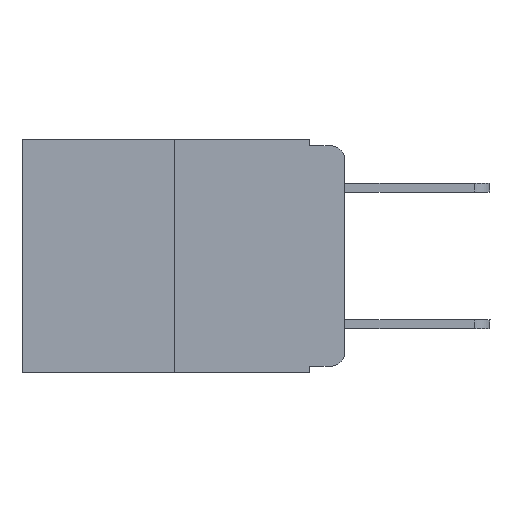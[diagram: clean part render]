
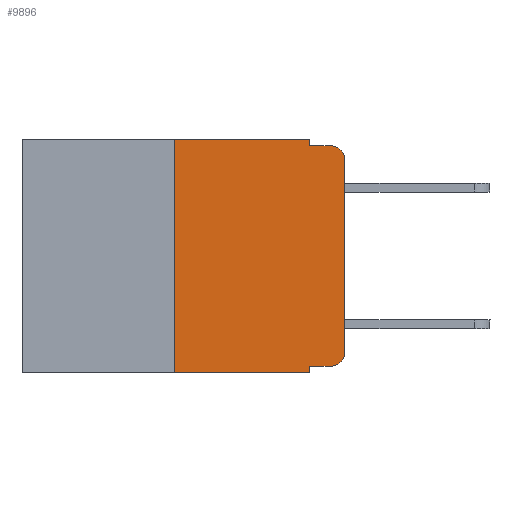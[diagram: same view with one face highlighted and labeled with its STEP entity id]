
A CAD part, left-side view. The second image highlights one B-rep face of the part: STEP entity #9896.
In plain terms, the highlighted planar face has unit normal (-1, 0, 0).
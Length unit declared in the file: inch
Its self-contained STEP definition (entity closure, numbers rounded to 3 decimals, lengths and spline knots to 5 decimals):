
#275 = LINE ( 'NONE', #21118, #16791 ) ;
#356 = DIRECTION ( 'NONE',  ( -1., 0., 0. ) ) ;
#552 = EDGE_CURVE ( 'NONE', #11415, #7567, #9098, .T. ) ;
#664 = DIRECTION ( 'NONE',  ( -1., 0., 0. ) ) ;
#775 = VERTEX_POINT ( 'NONE', #5129 ) ;
#997 = AXIS2_PLACEMENT_3D ( 'NONE', #3236, #20541, #8429 ) ;
#1747 = CARTESIAN_POINT ( 'NONE',  ( 0., 0., 0. ) ) ;
#1887 = DIRECTION ( 'NONE',  ( 0., 0., -1. ) ) ;
#2040 = VERTEX_POINT ( 'NONE', #16216 ) ;
#2120 = ORIENTED_EDGE ( 'NONE', *, *, #552, .T. ) ;
#2182 = CARTESIAN_POINT ( 'NONE',  ( 0., 0.473, -0.343 ) ) ;
#2504 = ORIENTED_EDGE ( 'NONE', *, *, #9815, .F. ) ;
#2686 = VECTOR ( 'NONE', #15383, 39.37008 ) ;
#2992 = CARTESIAN_POINT ( 'NONE',  ( 0., 0.473, 0. ) ) ;
#3052 = CARTESIAN_POINT ( 'NONE',  ( 0., 0.051, -0.01 ) ) ;
#3236 = CARTESIAN_POINT ( 'NONE',  ( 0., 0.473, 0. ) ) ;
#3288 = CARTESIAN_POINT ( 'NONE',  ( 0., 0.02, -0.333 ) ) ;
#3458 = VERTEX_POINT ( 'NONE', #17536 ) ;
#3771 = ORIENTED_EDGE ( 'NONE', *, *, #14911, .F. ) ;
#5129 = CARTESIAN_POINT ( 'NONE',  ( 0., 0.25, -0.343 ) ) ;
#5408 = VERTEX_POINT ( 'NONE', #13309 ) ;
#5728 = DIRECTION ( 'NONE',  ( 0., -1., 0. ) ) ;
#5820 = VECTOR ( 'NONE', #12043, 39.37008 ) ;
#6026 = ORIENTED_EDGE ( 'NONE', *, *, #7928, .T. ) ;
#7440 = DIRECTION ( 'NONE',  ( 0., 0., -1. ) ) ;
#7567 = VERTEX_POINT ( 'NONE', #14867 ) ;
#7669 = ORIENTED_EDGE ( 'NONE', *, *, #17644, .F. ) ;
#7928 = EDGE_CURVE ( 'NONE', #775, #10947, #13786, .T. ) ;
#8265 = CARTESIAN_POINT ( 'NONE',  ( 0., 0.051, 0. ) ) ;
#8429 = DIRECTION ( 'NONE',  ( 0., 0., -1. ) ) ;
#8486 = ORIENTED_EDGE ( 'NONE', *, *, #16528, .T. ) ;
#9098 = CIRCLE ( 'NONE', #13086, 0.02 ) ;
#9815 = EDGE_CURVE ( 'NONE', #775, #2040, #20059, .T. ) ;
#9896 = ADVANCED_FACE ( 'NONE', ( #22265 ), #11975, .F. ) ;
#10947 = VERTEX_POINT ( 'NONE', #14468 ) ;
#11323 = VECTOR ( 'NONE', #14043, 39.37008 ) ;
#11415 = VERTEX_POINT ( 'NONE', #14407 ) ;
#11485 = DIRECTION ( 'NONE',  ( 0., 0., -1. ) ) ;
#11516 = CARTESIAN_POINT ( 'NONE',  ( 0., 0.25, 0. ) ) ;
#11975 = PLANE ( 'NONE',  #997 ) ;
#12043 = DIRECTION ( 'NONE',  ( 0., 0., -1. ) ) ;
#12186 = VECTOR ( 'NONE', #5728, 39.37008 ) ;
#12619 = DIRECTION ( 'NONE',  ( 0., -1., 0. ) ) ;
#12682 = LINE ( 'NONE', #1747, #11323 ) ;
#12960 = ORIENTED_EDGE ( 'NONE', *, *, #16557, .T. ) ;
#13086 = AXIS2_PLACEMENT_3D ( 'NONE', #14498, #356, #1887 ) ;
#13309 = CARTESIAN_POINT ( 'NONE',  ( 0., 0.051, -0.01 ) ) ;
#13405 = DIRECTION ( 'NONE',  ( 0., 0., 1. ) ) ;
#13537 = VERTEX_POINT ( 'NONE', #20638 ) ;
#13786 = LINE ( 'NONE', #2182, #12186 ) ;
#13906 = CARTESIAN_POINT ( 'NONE',  ( 0., 0., -0.313 ) ) ;
#14043 = DIRECTION ( 'NONE',  ( 0., 0., 1. ) ) ;
#14078 = ORIENTED_EDGE ( 'NONE', *, *, #16243, .F. ) ;
#14108 = VECTOR ( 'NONE', #11485, 39.37008 ) ;
#14407 = CARTESIAN_POINT ( 'NONE',  ( 0., 0., -0.03 ) ) ;
#14468 = CARTESIAN_POINT ( 'NONE',  ( 0., 0.051, -0.343 ) ) ;
#14498 = CARTESIAN_POINT ( 'NONE',  ( 0., 0.02, -0.03 ) ) ;
#14867 = CARTESIAN_POINT ( 'NONE',  ( 0., 0.02, -0.01 ) ) ;
#14911 = EDGE_CURVE ( 'NONE', #13537, #10947, #15495, .T. ) ;
#15144 = VECTOR ( 'NONE', #22417, 39.37008 ) ;
#15383 = DIRECTION ( 'NONE',  ( 0., -1., 0. ) ) ;
#15495 = LINE ( 'NONE', #18696, #14108 ) ;
#15679 = CIRCLE ( 'NONE', #18794, 0.02 ) ;
#15683 = VECTOR ( 'NONE', #13405, 39.37008 ) ;
#16216 = CARTESIAN_POINT ( 'NONE',  ( 0., 0.25, 0. ) ) ;
#16243 = EDGE_CURVE ( 'NONE', #5408, #7567, #22029, .T. ) ;
#16528 = EDGE_CURVE ( 'NONE', #17841, #11415, #12682, .T. ) ;
#16557 = EDGE_CURVE ( 'NONE', #13537, #21076, #275, .T. ) ;
#16564 = EDGE_CURVE ( 'NONE', #21076, #17841, #15679, .T. ) ;
#16791 = VECTOR ( 'NONE', #12619, 39.37008 ) ;
#17536 = CARTESIAN_POINT ( 'NONE',  ( 0., 0.051, 0. ) ) ;
#17644 = EDGE_CURVE ( 'NONE', #2040, #3458, #18672, .T. ) ;
#17841 = VERTEX_POINT ( 'NONE', #13906 ) ;
#18672 = LINE ( 'NONE', #2992, #2686 ) ;
#18696 = CARTESIAN_POINT ( 'NONE',  ( 0., 0.051, 0. ) ) ;
#18794 = AXIS2_PLACEMENT_3D ( 'NONE', #20024, #664, #7440 ) ;
#19698 = ORIENTED_EDGE ( 'NONE', *, *, #16564, .T. ) ;
#19871 = LINE ( 'NONE', #8265, #5820 ) ;
#20024 = CARTESIAN_POINT ( 'NONE',  ( 0., 0.02, -0.313 ) ) ;
#20059 = LINE ( 'NONE', #11516, #15683 ) ;
#20541 = DIRECTION ( 'NONE',  ( 1., 0., 0. ) ) ;
#20638 = CARTESIAN_POINT ( 'NONE',  ( 0., 0.051, -0.333 ) ) ;
#21076 = VERTEX_POINT ( 'NONE', #3288 ) ;
#21118 = CARTESIAN_POINT ( 'NONE',  ( 0., 0.051, -0.333 ) ) ;
#21237 = EDGE_LOOP ( 'NONE', ( #8486, #2120, #14078, #22663, #7669, #2504, #6026, #3771, #12960, #19698 ) ) ;
#22029 = LINE ( 'NONE', #3052, #15144 ) ;
#22265 = FACE_OUTER_BOUND ( 'NONE', #21237, .T. ) ;
#22417 = DIRECTION ( 'NONE',  ( 0., -1., 0. ) ) ;
#22459 = EDGE_CURVE ( 'NONE', #3458, #5408, #19871, .T. ) ;
#22663 = ORIENTED_EDGE ( 'NONE', *, *, #22459, .F. ) ;
